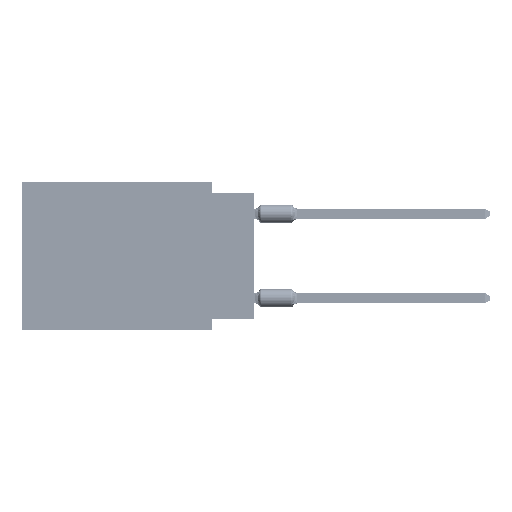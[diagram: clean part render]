
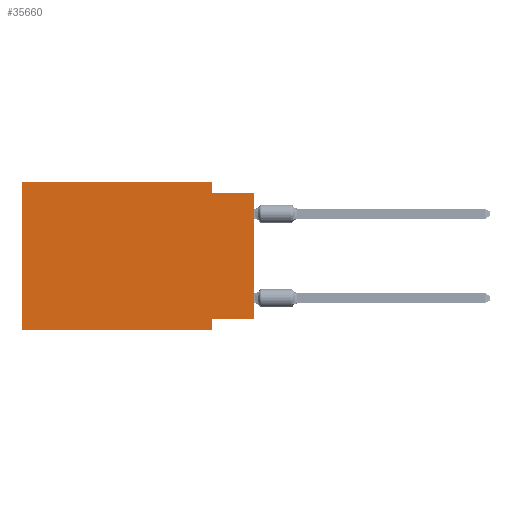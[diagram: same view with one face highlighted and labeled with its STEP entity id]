
A CAD part, left-side view. The second image highlights one B-rep face of the part: STEP entity #35660.
In plain terms, the highlighted planar face has unit normal (-1, 0, 0).
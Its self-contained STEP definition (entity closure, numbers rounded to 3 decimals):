
#416 = LINE ( 'NONE', #46899, #24439 ) ;
#523 = CARTESIAN_POINT ( 'NONE',  ( 0., 2.54, -8.255 ) ) ;
#1929 = EDGE_CURVE ( 'NONE', #61247, #51846, #5699, .T. ) ;
#3194 = LINE ( 'NONE', #65415, #63723 ) ;
#3830 = CARTESIAN_POINT ( 'NONE',  ( 0., 13.97, 0. ) ) ;
#5699 = LINE ( 'NONE', #26522, #62056 ) ;
#7943 = ORIENTED_EDGE ( 'NONE', *, *, #22380, .F. ) ;
#10739 = EDGE_LOOP ( 'NONE', ( #32652, #16856, #16398, #7943, #55683, #34812, #15200, #66224 ) ) ;
#11019 = CARTESIAN_POINT ( 'NONE',  ( 0., 2.54, -8.89 ) ) ;
#11264 = CARTESIAN_POINT ( 'NONE',  ( 0., 2.54, -0.635 ) ) ;
#12915 = AXIS2_PLACEMENT_3D ( 'NONE', #50513, #50174, #23514 ) ;
#13577 = CARTESIAN_POINT ( 'NONE',  ( 0., 13.97, -8.89 ) ) ;
#15200 = ORIENTED_EDGE ( 'NONE', *, *, #53906, .F. ) ;
#16398 = ORIENTED_EDGE ( 'NONE', *, *, #57342, .F. ) ;
#16729 = EDGE_CURVE ( 'NONE', #67286, #47833, #49379, .T. ) ;
#16751 = LINE ( 'NONE', #54326, #25987 ) ;
#16856 = ORIENTED_EDGE ( 'NONE', *, *, #16729, .F. ) ;
#16996 = EDGE_CURVE ( 'NONE', #37523, #44578, #16751, .T. ) ;
#18253 = DIRECTION ( 'NONE',  ( 0., -1., 0. ) ) ;
#21892 = LINE ( 'NONE', #26338, #55628 ) ;
#22380 = EDGE_CURVE ( 'NONE', #36714, #28712, #416, .T. ) ;
#23492 = EDGE_CURVE ( 'NONE', #37523, #36714, #3194, .T. ) ;
#23514 = DIRECTION ( 'NONE',  ( 0., 0., -1. ) ) ;
#24028 = DIRECTION ( 'NONE',  ( 0., 0., 1. ) ) ;
#24439 = VECTOR ( 'NONE', #66764, 1000. ) ;
#25987 = VECTOR ( 'NONE', #48198, 1000. ) ;
#26338 = CARTESIAN_POINT ( 'NONE',  ( 0., 2.54, -8.89 ) ) ;
#26522 = CARTESIAN_POINT ( 'NONE',  ( 0., 0., -8.255 ) ) ;
#28712 = VERTEX_POINT ( 'NONE', #53639 ) ;
#29320 = FACE_OUTER_BOUND ( 'NONE', #10739, .T. ) ;
#32652 = ORIENTED_EDGE ( 'NONE', *, *, #56287, .T. ) ;
#33623 = CARTESIAN_POINT ( 'NONE',  ( 0., 0., -0.635 ) ) ;
#33991 = CARTESIAN_POINT ( 'NONE',  ( 0., 0., -8.255 ) ) ;
#34812 = ORIENTED_EDGE ( 'NONE', *, *, #16996, .T. ) ;
#35660 = ADVANCED_FACE ( 'NONE', ( #29320 ), #60110, .F. ) ;
#36714 = VERTEX_POINT ( 'NONE', #3830 ) ;
#37523 = VERTEX_POINT ( 'NONE', #13577 ) ;
#37880 = CARTESIAN_POINT ( 'NONE',  ( 0., 0., 0. ) ) ;
#39629 = DIRECTION ( 'NONE',  ( 0., 0., -1. ) ) ;
#40299 = LINE ( 'NONE', #49888, #43925 ) ;
#41241 = DIRECTION ( 'NONE',  ( 0., 1., 0. ) ) ;
#42668 = LINE ( 'NONE', #37880, #54735 ) ;
#42748 = DIRECTION ( 'NONE',  ( 0., 0., -1. ) ) ;
#43925 = VECTOR ( 'NONE', #39629, 1000. ) ;
#44578 = VERTEX_POINT ( 'NONE', #11019 ) ;
#46899 = CARTESIAN_POINT ( 'NONE',  ( 0., 13.97, 0. ) ) ;
#47773 = VECTOR ( 'NONE', #18253, 1000. ) ;
#47833 = VERTEX_POINT ( 'NONE', #62819 ) ;
#48198 = DIRECTION ( 'NONE',  ( 0., -1., 0. ) ) ;
#49379 = LINE ( 'NONE', #33623, #47773 ) ;
#49888 = CARTESIAN_POINT ( 'NONE',  ( 0., 2.54, 0. ) ) ;
#50174 = DIRECTION ( 'NONE',  ( 1., 0., 0. ) ) ;
#50513 = CARTESIAN_POINT ( 'NONE',  ( 0., 13.97, 0. ) ) ;
#51846 = VERTEX_POINT ( 'NONE', #523 ) ;
#53639 = CARTESIAN_POINT ( 'NONE',  ( 0., 2.54, 0. ) ) ;
#53906 = EDGE_CURVE ( 'NONE', #51846, #44578, #21892, .T. ) ;
#54326 = CARTESIAN_POINT ( 'NONE',  ( 0., 13.97, -8.89 ) ) ;
#54735 = VECTOR ( 'NONE', #58743, 1000. ) ;
#55628 = VECTOR ( 'NONE', #42748, 1000. ) ;
#55683 = ORIENTED_EDGE ( 'NONE', *, *, #23492, .F. ) ;
#56287 = EDGE_CURVE ( 'NONE', #61247, #47833, #42668, .T. ) ;
#57342 = EDGE_CURVE ( 'NONE', #28712, #67286, #40299, .T. ) ;
#58743 = DIRECTION ( 'NONE',  ( 0., 0., 1. ) ) ;
#60110 = PLANE ( 'NONE',  #12915 ) ;
#61247 = VERTEX_POINT ( 'NONE', #33991 ) ;
#62056 = VECTOR ( 'NONE', #41241, 1000. ) ;
#62819 = CARTESIAN_POINT ( 'NONE',  ( 0., 0., -0.635 ) ) ;
#63723 = VECTOR ( 'NONE', #24028, 1000. ) ;
#65415 = CARTESIAN_POINT ( 'NONE',  ( 0., 13.97, 0. ) ) ;
#66224 = ORIENTED_EDGE ( 'NONE', *, *, #1929, .F. ) ;
#66764 = DIRECTION ( 'NONE',  ( 0., -1., 0. ) ) ;
#67286 = VERTEX_POINT ( 'NONE', #11264 ) ;
